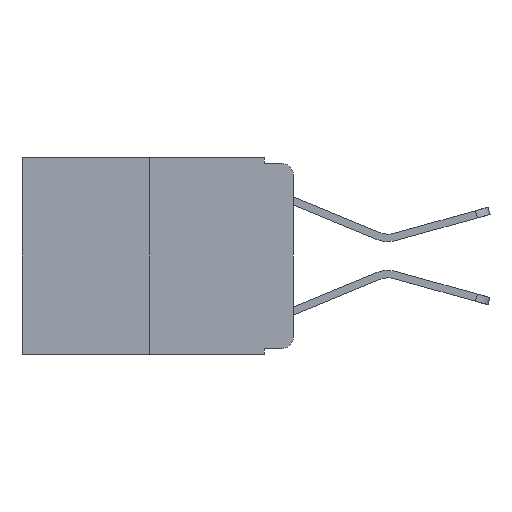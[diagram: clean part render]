
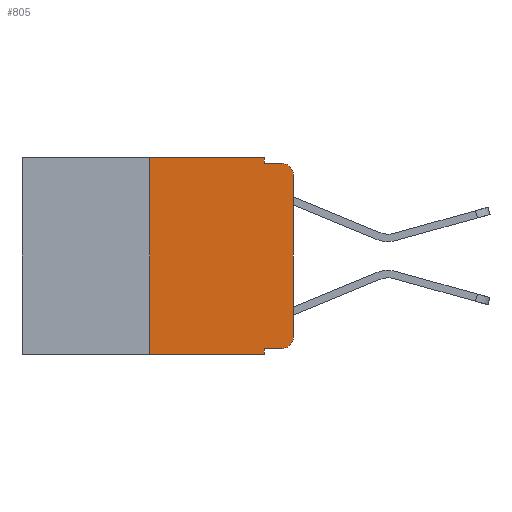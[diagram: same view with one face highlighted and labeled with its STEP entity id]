
A CAD part, left-side view. The second image highlights one B-rep face of the part: STEP entity #805.
In plain terms, the highlighted planar face has unit normal (-1, 0, 0).
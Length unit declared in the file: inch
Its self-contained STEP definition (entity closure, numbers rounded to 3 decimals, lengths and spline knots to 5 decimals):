
#221 = AXIS2_PLACEMENT_3D ( 'NONE', #5432, #6183, #3439 ) ;
#805 = ADVANCED_FACE ( 'NONE', ( #2166 ), #9796, .F. ) ;
#917 = EDGE_CURVE ( 'NONE', #6367, #6969, #8984, .T. ) ;
#1075 = EDGE_CURVE ( 'NONE', #9447, #6367, #5402, .T. ) ;
#1137 = EDGE_CURVE ( 'NONE', #1828, #1312, #2360, .T. ) ;
#1171 = VERTEX_POINT ( 'NONE', #5474 ) ;
#1178 = DIRECTION ( 'NONE',  ( 0., 0., 1. ) ) ;
#1248 = EDGE_CURVE ( 'NONE', #6782, #1828, #8512, .T. ) ;
#1262 = EDGE_CURVE ( 'NONE', #5948, #6782, #9916, .T. ) ;
#1280 = EDGE_CURVE ( 'NONE', #1171, #7513, #6596, .T. ) ;
#1284 = EDGE_CURVE ( 'NONE', #5948, #9314, #3859, .T. ) ;
#1302 = EDGE_CURVE ( 'NONE', #1312, #7513, #1551, .T. ) ;
#1304 = EDGE_CURVE ( 'NONE', #6969, #1171, #9545, .T. ) ;
#1312 = VERTEX_POINT ( 'NONE', #2357 ) ;
#1551 = CIRCLE ( 'NONE', #4575, 0.02 ) ;
#1630 = EDGE_CURVE ( 'NONE', #9447, #9314, #9537, .T. ) ;
#1679 = AXIS2_PLACEMENT_3D ( 'NONE', #6628, #8431, #9343 ) ;
#1768 = DIRECTION ( 'NONE',  ( 0., -1., 0. ) ) ;
#1828 = VERTEX_POINT ( 'NONE', #9426 ) ;
#2007 = CARTESIAN_POINT ( 'NONE',  ( 0., 0.051, -0.01 ) ) ;
#2166 = FACE_OUTER_BOUND ( 'NONE', #5430, .T. ) ;
#2206 = DIRECTION ( 'NONE',  ( 0., 0., -1. ) ) ;
#2357 = CARTESIAN_POINT ( 'NONE',  ( 0., 0., -0.03 ) ) ;
#2360 = LINE ( 'NONE', #4815, #4282 ) ;
#2426 = DIRECTION ( 'NONE',  ( 0., 0., 1. ) ) ;
#2579 = ORIENTED_EDGE ( 'NONE', *, *, #1302, .T. ) ;
#2689 = CARTESIAN_POINT ( 'NONE',  ( 0., 0.25, 0. ) ) ;
#2727 = CARTESIAN_POINT ( 'NONE',  ( 0., 0.051, 0. ) ) ;
#2737 = DIRECTION ( 'NONE',  ( 0., -1., 0. ) ) ;
#3161 = ORIENTED_EDGE ( 'NONE', *, *, #1137, .T. ) ;
#3439 = DIRECTION ( 'NONE',  ( 0., 0., -1. ) ) ;
#3538 = CARTESIAN_POINT ( 'NONE',  ( 0., 0.02, -0.01 ) ) ;
#3801 = ORIENTED_EDGE ( 'NONE', *, *, #1280, .F. ) ;
#3847 = VECTOR ( 'NONE', #5647, 39.37008 ) ;
#3859 = LINE ( 'NONE', #5912, #8096 ) ;
#4134 = VECTOR ( 'NONE', #1768, 39.37008 ) ;
#4282 = VECTOR ( 'NONE', #2426, 39.37008 ) ;
#4341 = CARTESIAN_POINT ( 'NONE',  ( 0., 0.051, -0.333 ) ) ;
#4351 = CARTESIAN_POINT ( 'NONE',  ( 0., 0.02, -0.03 ) ) ;
#4365 = DIRECTION ( 'NONE',  ( -1., 0., 0. ) ) ;
#4371 = DIRECTION ( 'NONE',  ( 0., 0., -1. ) ) ;
#4546 = ORIENTED_EDGE ( 'NONE', *, *, #1304, .F. ) ;
#4570 = ORIENTED_EDGE ( 'NONE', *, *, #917, .F. ) ;
#4575 = AXIS2_PLACEMENT_3D ( 'NONE', #4351, #4365, #4371 ) ;
#4587 = ORIENTED_EDGE ( 'NONE', *, *, #1075, .F. ) ;
#4815 = CARTESIAN_POINT ( 'NONE',  ( 0., 0., 0. ) ) ;
#4998 = CARTESIAN_POINT ( 'NONE',  ( 0., 0.473, 0. ) ) ;
#5081 = VECTOR ( 'NONE', #2737, 39.37008 ) ;
#5253 = CARTESIAN_POINT ( 'NONE',  ( 0., 0.051, -0.343 ) ) ;
#5402 = LINE ( 'NONE', #5840, #9007 ) ;
#5430 = EDGE_LOOP ( 'NONE', ( #3161, #2579, #3801, #4546, #4570, #4587, #5740, #6633, #5681, #5770 ) ) ;
#5432 = CARTESIAN_POINT ( 'NONE',  ( 0., 0.473, 0. ) ) ;
#5474 = CARTESIAN_POINT ( 'NONE',  ( 0., 0.051, -0.01 ) ) ;
#5647 = DIRECTION ( 'NONE',  ( 0., -1., 0. ) ) ;
#5681 = ORIENTED_EDGE ( 'NONE', *, *, #1262, .T. ) ;
#5740 = ORIENTED_EDGE ( 'NONE', *, *, #1630, .T. ) ;
#5770 = ORIENTED_EDGE ( 'NONE', *, *, #1248, .T. ) ;
#5840 = CARTESIAN_POINT ( 'NONE',  ( 0., 0.25, 0. ) ) ;
#5884 = VECTOR ( 'NONE', #2206, 39.37008 ) ;
#5912 = CARTESIAN_POINT ( 'NONE',  ( 0., 0.051, 0. ) ) ;
#5948 = VERTEX_POINT ( 'NONE', #4341 ) ;
#5976 = DIRECTION ( 'NONE',  ( 0., 0., -1. ) ) ;
#6183 = DIRECTION ( 'NONE',  ( 1., 0., 0. ) ) ;
#6367 = VERTEX_POINT ( 'NONE', #2689 ) ;
#6431 = CARTESIAN_POINT ( 'NONE',  ( 0., 0.02, -0.333 ) ) ;
#6545 = DIRECTION ( 'NONE',  ( 0., -1., 0. ) ) ;
#6596 = LINE ( 'NONE', #2007, #4134 ) ;
#6623 = CARTESIAN_POINT ( 'NONE',  ( 0., 0.051, -0.333 ) ) ;
#6628 = CARTESIAN_POINT ( 'NONE',  ( 0., 0.02, -0.313 ) ) ;
#6633 = ORIENTED_EDGE ( 'NONE', *, *, #1284, .F. ) ;
#6782 = VERTEX_POINT ( 'NONE', #6431 ) ;
#6969 = VERTEX_POINT ( 'NONE', #9223 ) ;
#6990 = CARTESIAN_POINT ( 'NONE',  ( 0., 0.473, -0.343 ) ) ;
#7513 = VERTEX_POINT ( 'NONE', #3538 ) ;
#8096 = VECTOR ( 'NONE', #5976, 39.37008 ) ;
#8311 = VECTOR ( 'NONE', #6545, 39.37008 ) ;
#8335 = CARTESIAN_POINT ( 'NONE',  ( 0., 0.25, -0.343 ) ) ;
#8431 = DIRECTION ( 'NONE',  ( -1., 0., 0. ) ) ;
#8512 = CIRCLE ( 'NONE', #1679, 0.02 ) ;
#8984 = LINE ( 'NONE', #4998, #5081 ) ;
#9007 = VECTOR ( 'NONE', #1178, 39.37008 ) ;
#9223 = CARTESIAN_POINT ( 'NONE',  ( 0., 0.051, 0. ) ) ;
#9314 = VERTEX_POINT ( 'NONE', #5253 ) ;
#9343 = DIRECTION ( 'NONE',  ( 0., 0., -1. ) ) ;
#9426 = CARTESIAN_POINT ( 'NONE',  ( 0., 0., -0.313 ) ) ;
#9447 = VERTEX_POINT ( 'NONE', #8335 ) ;
#9537 = LINE ( 'NONE', #6990, #3847 ) ;
#9545 = LINE ( 'NONE', #2727, #5884 ) ;
#9796 = PLANE ( 'NONE',  #221 ) ;
#9916 = LINE ( 'NONE', #6623, #8311 ) ;
